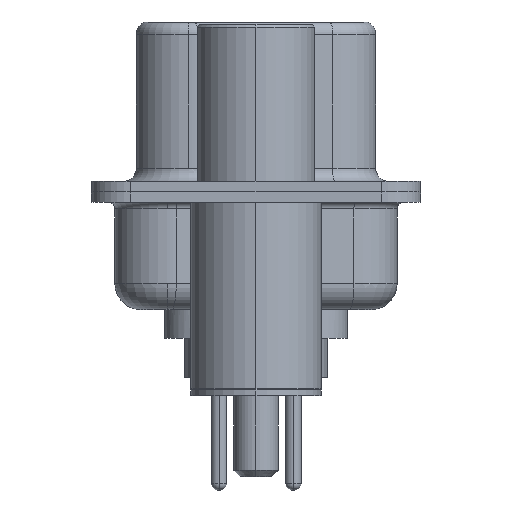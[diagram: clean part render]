
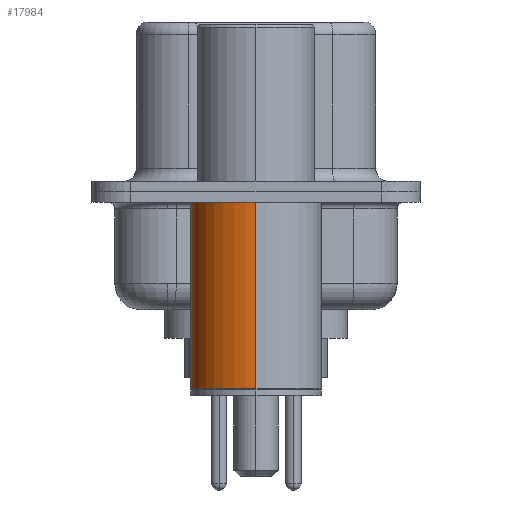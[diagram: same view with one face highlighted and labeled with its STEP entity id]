
A CAD part, left-side view. The second image highlights one B-rep face of the part: STEP entity #17984.
In plain terms, the highlighted cylindrical face has radius 2.5 mm (diameter 5 mm), a partial arc.
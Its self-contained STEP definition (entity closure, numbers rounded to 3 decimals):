
#638 = CARTESIAN_POINT ( 'NONE',  ( -2.5, 0., 0.581 ) ) ;
#1931 = DIRECTION ( 'NONE',  ( 1., 0., 0. ) ) ;
#2376 = ORIENTED_EDGE ( 'NONE', *, *, #6135, .F. ) ;
#2494 = EDGE_LOOP ( 'NONE', ( #5453, #10165, #2376, #11081 ) ) ;
#2656 = LINE ( 'NONE', #638, #6563 ) ;
#2816 = VERTEX_POINT ( 'NONE', #11353 ) ;
#3322 = DIRECTION ( 'NONE',  ( 1., 0., 0. ) ) ;
#3433 = CARTESIAN_POINT ( 'NONE',  ( 0., 0., -0.4 ) ) ;
#3716 = AXIS2_PLACEMENT_3D ( 'NONE', #15776, #12324, #3322 ) ;
#3791 = EDGE_CURVE ( 'NONE', #16422, #2816, #7571, .T. ) ;
#3997 = DIRECTION ( 'NONE',  ( 0., 0., 1. ) ) ;
#4187 = VECTOR ( 'NONE', #11622, 1000. ) ;
#5076 = LINE ( 'NONE', #13071, #4187 ) ;
#5453 = ORIENTED_EDGE ( 'NONE', *, *, #3791, .T. ) ;
#6135 = EDGE_CURVE ( 'NONE', #12854, #11635, #16000, .T. ) ;
#6563 = VECTOR ( 'NONE', #3997, 1000. ) ;
#7139 = EDGE_CURVE ( 'NONE', #2816, #11635, #2656, .T. ) ;
#7571 = CIRCLE ( 'NONE', #3716, 2.5 ) ;
#7734 = DIRECTION ( 'NONE',  ( 1., 0., 0. ) ) ;
#9211 = CARTESIAN_POINT ( 'NONE',  ( 0., 0., 0.581 ) ) ;
#9723 = FACE_OUTER_BOUND ( 'NONE', #2494, .T. ) ;
#10165 = ORIENTED_EDGE ( 'NONE', *, *, #7139, .T. ) ;
#11081 = ORIENTED_EDGE ( 'NONE', *, *, #18311, .F. ) ;
#11353 = CARTESIAN_POINT ( 'NONE',  ( -2.5, 0., -7.525 ) ) ;
#11622 = DIRECTION ( 'NONE',  ( 0., 0., 1. ) ) ;
#11635 = VERTEX_POINT ( 'NONE', #12584 ) ;
#12324 = DIRECTION ( 'NONE',  ( 0., 0., 1. ) ) ;
#12584 = CARTESIAN_POINT ( 'NONE',  ( -2.5, 0., -0.4 ) ) ;
#12740 = CARTESIAN_POINT ( 'NONE',  ( 2.5, 0., -0.4 ) ) ;
#12854 = VERTEX_POINT ( 'NONE', #12740 ) ;
#13071 = CARTESIAN_POINT ( 'NONE',  ( 2.5, 0., 0.581 ) ) ;
#14592 = DIRECTION ( 'NONE',  ( 0., 0., 1. ) ) ;
#15536 = AXIS2_PLACEMENT_3D ( 'NONE', #9211, #16525, #7734 ) ;
#15776 = CARTESIAN_POINT ( 'NONE',  ( 0., 0., -7.525 ) ) ;
#16000 = CIRCLE ( 'NONE', #18544, 2.5 ) ;
#16422 = VERTEX_POINT ( 'NONE', #17575 ) ;
#16525 = DIRECTION ( 'NONE',  ( 0., 0., 1. ) ) ;
#17068 = CYLINDRICAL_SURFACE ( 'NONE', #15536, 2.5 ) ;
#17575 = CARTESIAN_POINT ( 'NONE',  ( 2.5, 0., -7.525 ) ) ;
#17984 = ADVANCED_FACE ( 'NONE', ( #9723 ), #17068, .T. ) ;
#18311 = EDGE_CURVE ( 'NONE', #16422, #12854, #5076, .T. ) ;
#18544 = AXIS2_PLACEMENT_3D ( 'NONE', #3433, #14592, #1931 ) ;
